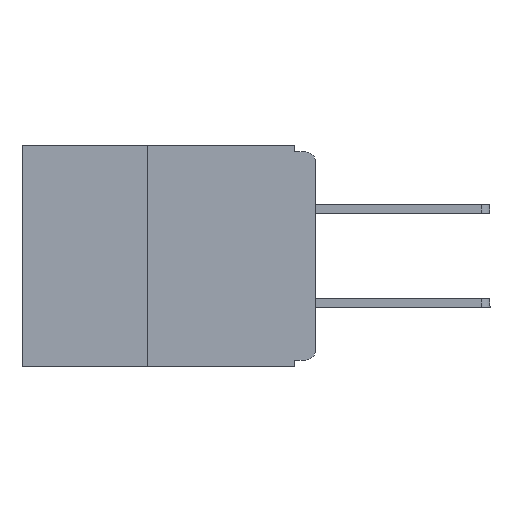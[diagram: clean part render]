
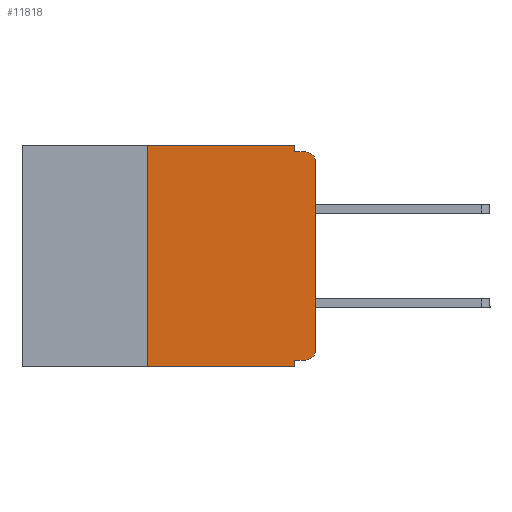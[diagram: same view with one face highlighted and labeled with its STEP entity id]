
A CAD part, left-side view. The second image highlights one B-rep face of the part: STEP entity #11818.
In plain terms, the highlighted planar face has unit normal (-1, 0, 0).
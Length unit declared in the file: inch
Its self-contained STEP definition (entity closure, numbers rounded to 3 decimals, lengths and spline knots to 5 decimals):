
#6 = ORIENTED_EDGE ( 'NONE', *, *, #10471, .T. ) ;
#128 = CARTESIAN_POINT ( 'NONE',  ( 0., 0.437, -0.33 ) ) ;
#142 = DIRECTION ( 'NONE',  ( 0., -1., 0. ) ) ;
#407 = EDGE_CURVE ( 'NONE', #11282, #7878, #1716, .T. ) ;
#884 = VECTOR ( 'NONE', #8875, 39.37008 ) ;
#982 = VECTOR ( 'NONE', #4375, 39.37008 ) ;
#988 = CARTESIAN_POINT ( 'NONE',  ( 0., 0.031, -0.01 ) ) ;
#1228 = CARTESIAN_POINT ( 'NONE',  ( 0., 0., -0.01 ) ) ;
#1434 = ORIENTED_EDGE ( 'NONE', *, *, #4998, .F. ) ;
#1462 = LINE ( 'NONE', #6900, #10037 ) ;
#1584 = LINE ( 'NONE', #7752, #884 ) ;
#1600 = VERTEX_POINT ( 'NONE', #8912 ) ;
#1652 = LINE ( 'NONE', #4531, #13084 ) ;
#1716 = LINE ( 'NONE', #128, #2064 ) ;
#1958 = ORIENTED_EDGE ( 'NONE', *, *, #8180, .F. ) ;
#2064 = VECTOR ( 'NONE', #142, 39.37008 ) ;
#2173 = CIRCLE ( 'NONE', #4429, 0.015 ) ;
#2379 = VERTEX_POINT ( 'NONE', #4449 ) ;
#2502 = ORIENTED_EDGE ( 'NONE', *, *, #407, .T. ) ;
#2641 = PLANE ( 'NONE',  #8738 ) ;
#2842 = ORIENTED_EDGE ( 'NONE', *, *, #13484, .F. ) ;
#3583 = CARTESIAN_POINT ( 'NONE',  ( 0., 0.25, -0.33 ) ) ;
#3815 = DIRECTION ( 'NONE',  ( 0., 1., 0. ) ) ;
#4053 = EDGE_CURVE ( 'NONE', #1600, #2379, #5642, .T. ) ;
#4137 = CARTESIAN_POINT ( 'NONE',  ( 0., 0., 0. ) ) ;
#4184 = EDGE_CURVE ( 'NONE', #11282, #12732, #7235, .T. ) ;
#4375 = DIRECTION ( 'NONE',  ( 0., 0., 1. ) ) ;
#4429 = AXIS2_PLACEMENT_3D ( 'NONE', #4870, #12667, #6002 ) ;
#4449 = CARTESIAN_POINT ( 'NONE',  ( 0., 0., -0.025 ) ) ;
#4531 = CARTESIAN_POINT ( 'NONE',  ( 0., 0., -0.32 ) ) ;
#4785 = CARTESIAN_POINT ( 'NONE',  ( 0., 0.015, -0.32 ) ) ;
#4825 = DIRECTION ( 'NONE',  ( 0., 0., -1. ) ) ;
#4870 = CARTESIAN_POINT ( 'NONE',  ( 0., 0.015, -0.305 ) ) ;
#4998 = EDGE_CURVE ( 'NONE', #7759, #5639, #8288, .T. ) ;
#5012 = ORIENTED_EDGE ( 'NONE', *, *, #12265, .F. ) ;
#5059 = EDGE_CURVE ( 'NONE', #7744, #10773, #1652, .T. ) ;
#5165 = CARTESIAN_POINT ( 'NONE',  ( 0., 0.031, 0. ) ) ;
#5215 = DIRECTION ( 'NONE',  ( 0., 0., -1. ) ) ;
#5258 = DIRECTION ( 'NONE',  ( 0., 0., 1. ) ) ;
#5269 = VECTOR ( 'NONE', #5215, 39.37008 ) ;
#5481 = CARTESIAN_POINT ( 'NONE',  ( 0., 0.015, -0.025 ) ) ;
#5639 = VERTEX_POINT ( 'NONE', #988 ) ;
#5640 = FACE_OUTER_BOUND ( 'NONE', #8331, .T. ) ;
#5642 = LINE ( 'NONE', #4137, #14121 ) ;
#5766 = DIRECTION ( 'NONE',  ( 0., 0., -1. ) ) ;
#5950 = EDGE_CURVE ( 'NONE', #7744, #1600, #2173, .T. ) ;
#6002 = DIRECTION ( 'NONE',  ( 0., 0., -1. ) ) ;
#6296 = CARTESIAN_POINT ( 'NONE',  ( 0., 0.25, -0.33 ) ) ;
#6419 = ORIENTED_EDGE ( 'NONE', *, *, #4053, .T. ) ;
#6600 = DIRECTION ( 'NONE',  ( 0., 0., -1. ) ) ;
#6900 = CARTESIAN_POINT ( 'NONE',  ( 0., 0.031, -0.33 ) ) ;
#7147 = CARTESIAN_POINT ( 'NONE',  ( 0., 0.031, -0.32 ) ) ;
#7235 = LINE ( 'NONE', #6296, #982 ) ;
#7622 = CARTESIAN_POINT ( 'NONE',  ( 0., 0.25, 0. ) ) ;
#7744 = VERTEX_POINT ( 'NONE', #4785 ) ;
#7752 = CARTESIAN_POINT ( 'NONE',  ( 0., 0.437, 0. ) ) ;
#7759 = VERTEX_POINT ( 'NONE', #13651 ) ;
#7878 = VERTEX_POINT ( 'NONE', #11682 ) ;
#8180 = EDGE_CURVE ( 'NONE', #12732, #7759, #1584, .T. ) ;
#8288 = LINE ( 'NONE', #5165, #5269 ) ;
#8331 = EDGE_LOOP ( 'NONE', ( #6419, #6, #5012, #1434, #1958, #9658, #2502, #2842, #9865, #9337 ) ) ;
#8649 = VECTOR ( 'NONE', #11257, 39.37008 ) ;
#8738 = AXIS2_PLACEMENT_3D ( 'NONE', #10456, #11548, #4825 ) ;
#8875 = DIRECTION ( 'NONE',  ( 0., -1., 0. ) ) ;
#8912 = CARTESIAN_POINT ( 'NONE',  ( 0., 0., -0.305 ) ) ;
#9237 = CARTESIAN_POINT ( 'NONE',  ( 0., 0.015, -0.01 ) ) ;
#9337 = ORIENTED_EDGE ( 'NONE', *, *, #5950, .T. ) ;
#9658 = ORIENTED_EDGE ( 'NONE', *, *, #4184, .F. ) ;
#9865 = ORIENTED_EDGE ( 'NONE', *, *, #5059, .F. ) ;
#10037 = VECTOR ( 'NONE', #5766, 39.37008 ) ;
#10132 = CIRCLE ( 'NONE', #13750, 0.015 ) ;
#10456 = CARTESIAN_POINT ( 'NONE',  ( 0., 0.437, 0. ) ) ;
#10471 = EDGE_CURVE ( 'NONE', #2379, #10650, #10132, .T. ) ;
#10650 = VERTEX_POINT ( 'NONE', #9237 ) ;
#10773 = VERTEX_POINT ( 'NONE', #7147 ) ;
#11257 = DIRECTION ( 'NONE',  ( 0., -1., 0. ) ) ;
#11282 = VERTEX_POINT ( 'NONE', #3583 ) ;
#11548 = DIRECTION ( 'NONE',  ( 1., 0., 0. ) ) ;
#11589 = LINE ( 'NONE', #1228, #8649 ) ;
#11682 = CARTESIAN_POINT ( 'NONE',  ( 0., 0.031, -0.33 ) ) ;
#11818 = ADVANCED_FACE ( 'NONE', ( #5640 ), #2641, .F. ) ;
#12265 = EDGE_CURVE ( 'NONE', #5639, #10650, #11589, .T. ) ;
#12667 = DIRECTION ( 'NONE',  ( -1., 0., 0. ) ) ;
#12732 = VERTEX_POINT ( 'NONE', #7622 ) ;
#13084 = VECTOR ( 'NONE', #3815, 39.37008 ) ;
#13246 = DIRECTION ( 'NONE',  ( -1., 0., 0. ) ) ;
#13484 = EDGE_CURVE ( 'NONE', #10773, #7878, #1462, .T. ) ;
#13651 = CARTESIAN_POINT ( 'NONE',  ( 0., 0.031, 0. ) ) ;
#13750 = AXIS2_PLACEMENT_3D ( 'NONE', #5481, #13246, #6600 ) ;
#14121 = VECTOR ( 'NONE', #5258, 39.37008 ) ;
